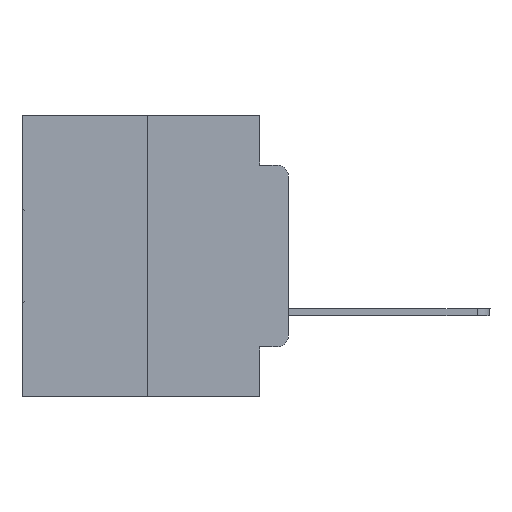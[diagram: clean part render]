
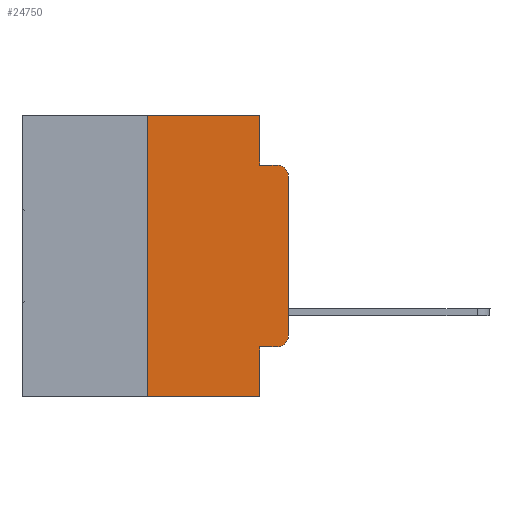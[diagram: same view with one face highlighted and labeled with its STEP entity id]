
A CAD part, left-side view. The second image highlights one B-rep face of the part: STEP entity #24750.
In plain terms, the highlighted planar face has unit normal (-1, 0, 0).
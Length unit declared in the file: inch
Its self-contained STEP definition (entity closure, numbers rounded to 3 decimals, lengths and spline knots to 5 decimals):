
#116 = LINE ( 'NONE', #3188, #15127 ) ;
#245 = CIRCLE ( 'NONE', #19241, 0.02 ) ;
#466 = CARTESIAN_POINT ( 'NONE',  ( 0., 0.02, -0.3915 ) ) ;
#583 = EDGE_LOOP ( 'NONE', ( #28628, #5897, #8695, #3261, #7883, #1881, #24312, #11718, #13521, #10521 ) ) ;
#1180 = DIRECTION ( 'NONE',  ( 0., 0., 1. ) ) ;
#1609 = VERTEX_POINT ( 'NONE', #19217 ) ;
#1686 = DIRECTION ( 'NONE',  ( 0., 0., -1. ) ) ;
#1848 = VERTEX_POINT ( 'NONE', #5313 ) ;
#1866 = CARTESIAN_POINT ( 'NONE',  ( 0., 0.051, -0.5 ) ) ;
#1881 = ORIENTED_EDGE ( 'NONE', *, *, #10701, .F. ) ;
#2059 = DIRECTION ( 'NONE',  ( 0., -1., 0. ) ) ;
#2285 = CARTESIAN_POINT ( 'NONE',  ( 0., 0.051, -0.0885 ) ) ;
#3003 = VECTOR ( 'NONE', #1180, 39.37008 ) ;
#3188 = CARTESIAN_POINT ( 'NONE',  ( 0., 0.051, 0. ) ) ;
#3261 = ORIENTED_EDGE ( 'NONE', *, *, #17801, .F. ) ;
#3277 = LINE ( 'NONE', #7384, #11949 ) ;
#3401 = CARTESIAN_POINT ( 'NONE',  ( 0., 0.473, -0.5 ) ) ;
#3990 = CARTESIAN_POINT ( 'NONE',  ( 0., 0.051, 0. ) ) ;
#4092 = EDGE_CURVE ( 'NONE', #1848, #11618, #26628, .T. ) ;
#4707 = VERTEX_POINT ( 'NONE', #8326 ) ;
#5313 = CARTESIAN_POINT ( 'NONE',  ( 0., 0., -0.3915 ) ) ;
#5897 = ORIENTED_EDGE ( 'NONE', *, *, #12205, .T. ) ;
#5972 = CARTESIAN_POINT ( 'NONE',  ( 0., 0.02, -0.1085 ) ) ;
#6079 = AXIS2_PLACEMENT_3D ( 'NONE', #6741, #25638, #23357 ) ;
#6289 = DIRECTION ( 'NONE',  ( 0., -1., 0. ) ) ;
#6723 = VECTOR ( 'NONE', #27849, 39.37008 ) ;
#6741 = CARTESIAN_POINT ( 'NONE',  ( 0., 0.473, 0. ) ) ;
#6885 = PLANE ( 'NONE',  #6079 ) ;
#7350 = EDGE_CURVE ( 'NONE', #8110, #14762, #3277, .T. ) ;
#7384 = CARTESIAN_POINT ( 'NONE',  ( 0., 0.473, 0. ) ) ;
#7500 = DIRECTION ( 'NONE',  ( 0., 0., -1. ) ) ;
#7551 = CARTESIAN_POINT ( 'NONE',  ( 0., 0., -0.1085 ) ) ;
#7858 = EDGE_CURVE ( 'NONE', #25108, #1848, #245, .T. ) ;
#7883 = ORIENTED_EDGE ( 'NONE', *, *, #7350, .F. ) ;
#8110 = VERTEX_POINT ( 'NONE', #27565 ) ;
#8326 = CARTESIAN_POINT ( 'NONE',  ( 0., 0.051, -0.0885 ) ) ;
#8584 = CARTESIAN_POINT ( 'NONE',  ( 0., 0.25, -0.5 ) ) ;
#8695 = ORIENTED_EDGE ( 'NONE', *, *, #15339, .F. ) ;
#9190 = VERTEX_POINT ( 'NONE', #8584 ) ;
#10521 = ORIENTED_EDGE ( 'NONE', *, *, #7858, .T. ) ;
#10701 = EDGE_CURVE ( 'NONE', #9190, #8110, #11637, .T. ) ;
#10869 = LINE ( 'NONE', #3401, #24072 ) ;
#11339 = FACE_OUTER_BOUND ( 'NONE', #583, .T. ) ;
#11618 = VERTEX_POINT ( 'NONE', #7551 ) ;
#11637 = LINE ( 'NONE', #23193, #27420 ) ;
#11718 = ORIENTED_EDGE ( 'NONE', *, *, #18730, .F. ) ;
#11949 = VECTOR ( 'NONE', #28390, 39.37008 ) ;
#12193 = DIRECTION ( 'NONE',  ( 0., 0., -1. ) ) ;
#12205 = EDGE_CURVE ( 'NONE', #11618, #1609, #16333, .T. ) ;
#13254 = VECTOR ( 'NONE', #2059, 39.37008 ) ;
#13521 = ORIENTED_EDGE ( 'NONE', *, *, #22094, .T. ) ;
#13669 = LINE ( 'NONE', #22927, #13254 ) ;
#14174 = LINE ( 'NONE', #2285, #6723 ) ;
#14762 = VERTEX_POINT ( 'NONE', #3990 ) ;
#14772 = VERTEX_POINT ( 'NONE', #1866 ) ;
#15127 = VECTOR ( 'NONE', #12193, 39.37008 ) ;
#15339 = EDGE_CURVE ( 'NONE', #4707, #1609, #14174, .T. ) ;
#16333 = CIRCLE ( 'NONE', #17326, 0.02 ) ;
#17326 = AXIS2_PLACEMENT_3D ( 'NONE', #5972, #24992, #1686 ) ;
#17496 = CARTESIAN_POINT ( 'NONE',  ( 0., 0., 0. ) ) ;
#17801 = EDGE_CURVE ( 'NONE', #14762, #4707, #29544, .T. ) ;
#18290 = CARTESIAN_POINT ( 'NONE',  ( 0., 0.051, 0. ) ) ;
#18730 = EDGE_CURVE ( 'NONE', #22301, #14772, #116, .T. ) ;
#19217 = CARTESIAN_POINT ( 'NONE',  ( 0., 0.02, -0.0885 ) ) ;
#19241 = AXIS2_PLACEMENT_3D ( 'NONE', #466, #21672, #7500 ) ;
#20761 = DIRECTION ( 'NONE',  ( 0., 0., 1. ) ) ;
#21672 = DIRECTION ( 'NONE',  ( -1., 0., 0. ) ) ;
#22094 = EDGE_CURVE ( 'NONE', #22301, #25108, #13669, .T. ) ;
#22301 = VERTEX_POINT ( 'NONE', #27028 ) ;
#22927 = CARTESIAN_POINT ( 'NONE',  ( 0., 0.051, -0.4115 ) ) ;
#23193 = CARTESIAN_POINT ( 'NONE',  ( 0., 0.25, 0. ) ) ;
#23357 = DIRECTION ( 'NONE',  ( 0., 0., -1. ) ) ;
#24072 = VECTOR ( 'NONE', #6289, 39.37008 ) ;
#24257 = CARTESIAN_POINT ( 'NONE',  ( 0., 0.02, -0.4115 ) ) ;
#24312 = ORIENTED_EDGE ( 'NONE', *, *, #29610, .T. ) ;
#24750 = ADVANCED_FACE ( 'NONE', ( #11339 ), #6885, .F. ) ;
#24992 = DIRECTION ( 'NONE',  ( -1., 0., 0. ) ) ;
#25090 = VECTOR ( 'NONE', #25277, 39.37008 ) ;
#25108 = VERTEX_POINT ( 'NONE', #24257 ) ;
#25277 = DIRECTION ( 'NONE',  ( 0., 0., -1. ) ) ;
#25638 = DIRECTION ( 'NONE',  ( 1., 0., 0. ) ) ;
#26628 = LINE ( 'NONE', #17496, #3003 ) ;
#27028 = CARTESIAN_POINT ( 'NONE',  ( 0., 0.051, -0.4115 ) ) ;
#27420 = VECTOR ( 'NONE', #20761, 39.37008 ) ;
#27565 = CARTESIAN_POINT ( 'NONE',  ( 0., 0.25, 0. ) ) ;
#27849 = DIRECTION ( 'NONE',  ( 0., -1., 0. ) ) ;
#28390 = DIRECTION ( 'NONE',  ( 0., -1., 0. ) ) ;
#28628 = ORIENTED_EDGE ( 'NONE', *, *, #4092, .T. ) ;
#29544 = LINE ( 'NONE', #18290, #25090 ) ;
#29610 = EDGE_CURVE ( 'NONE', #9190, #14772, #10869, .T. ) ;
